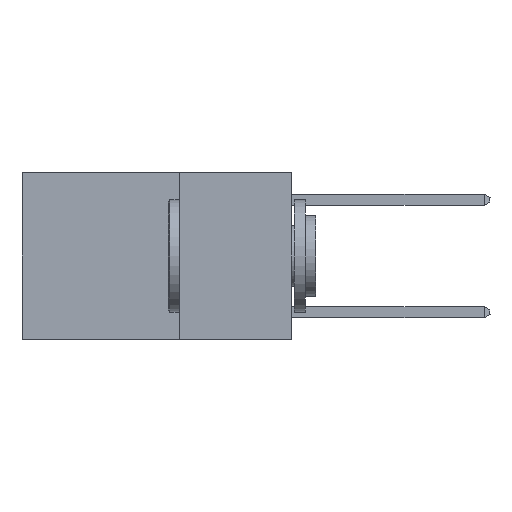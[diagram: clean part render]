
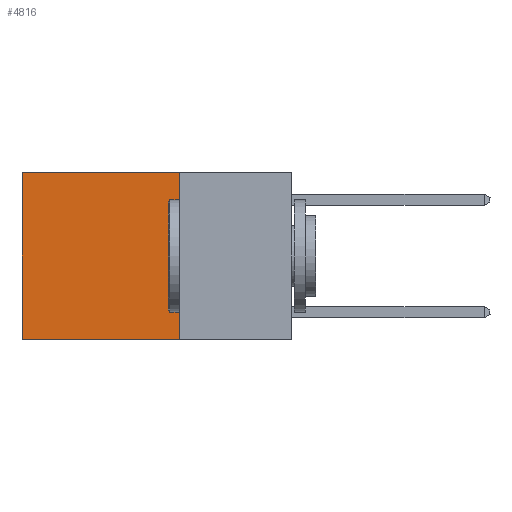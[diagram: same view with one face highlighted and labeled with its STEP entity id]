
A CAD part, left-side view. The second image highlights one B-rep face of the part: STEP entity #4816.
In plain terms, the highlighted planar face has unit normal (-1, 0, 0).
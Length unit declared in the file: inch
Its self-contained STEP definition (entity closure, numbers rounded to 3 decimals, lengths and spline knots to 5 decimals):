
#78 = LINE ( 'NONE', #3020, #11518 ) ;
#311 = CARTESIAN_POINT ( 'NONE',  ( 0.2625, 0.25, 0. ) ) ;
#857 = EDGE_CURVE ( 'NONE', #5635, #7671, #12639, .T. ) ;
#1300 = DIRECTION ( 'NONE',  ( 0., 0., -1. ) ) ;
#1972 = DIRECTION ( 'NONE',  ( 0., 0., -1. ) ) ;
#2301 = EDGE_LOOP ( 'NONE', ( #2913, #7093, #7404, #3521 ) ) ;
#2913 = ORIENTED_EDGE ( 'NONE', *, *, #4659, .T. ) ;
#3020 = CARTESIAN_POINT ( 'NONE',  ( 0.2625, 0.25, -0.37 ) ) ;
#3116 = CARTESIAN_POINT ( 'NONE',  ( 0.2625, 0.6, -0.37 ) ) ;
#3497 = VECTOR ( 'NONE', #10661, 39.37008 ) ;
#3521 = ORIENTED_EDGE ( 'NONE', *, *, #857, .T. ) ;
#4631 = DIRECTION ( 'NONE',  ( 1., 0., 0. ) ) ;
#4659 = EDGE_CURVE ( 'NONE', #7671, #6860, #12641, .T. ) ;
#4816 = ADVANCED_FACE ( 'NONE', ( #8830 ), #9019, .F. ) ;
#4895 = CARTESIAN_POINT ( 'NONE',  ( 0.2625, 0.25, -0.37 ) ) ;
#5111 = VECTOR ( 'NONE', #1972, 39.37008 ) ;
#5118 = LINE ( 'NONE', #9227, #5111 ) ;
#5635 = VERTEX_POINT ( 'NONE', #311 ) ;
#6021 = EDGE_CURVE ( 'NONE', #11185, #6860, #78, .T. ) ;
#6753 = DIRECTION ( 'NONE',  ( 0., 0., -1. ) ) ;
#6860 = VERTEX_POINT ( 'NONE', #3116 ) ;
#7093 = ORIENTED_EDGE ( 'NONE', *, *, #6021, .F. ) ;
#7309 = DIRECTION ( 'NONE',  ( 0., 1., 0. ) ) ;
#7404 = ORIENTED_EDGE ( 'NONE', *, *, #12106, .F. ) ;
#7671 = VERTEX_POINT ( 'NONE', #9993 ) ;
#7755 = CARTESIAN_POINT ( 'NONE',  ( 0.2625, 0.25, 0. ) ) ;
#8830 = FACE_OUTER_BOUND ( 'NONE', #2301, .T. ) ;
#9019 = PLANE ( 'NONE',  #9957 ) ;
#9227 = CARTESIAN_POINT ( 'NONE',  ( 0.2625, 0.25, 0. ) ) ;
#9511 = CARTESIAN_POINT ( 'NONE',  ( 0.2625, 0.6, 0. ) ) ;
#9957 = AXIS2_PLACEMENT_3D ( 'NONE', #7755, #4631, #6753 ) ;
#9993 = CARTESIAN_POINT ( 'NONE',  ( 0.2625, 0.6, 0. ) ) ;
#10661 = DIRECTION ( 'NONE',  ( 0., 1., 0. ) ) ;
#10730 = VECTOR ( 'NONE', #1300, 39.37008 ) ;
#11185 = VERTEX_POINT ( 'NONE', #4895 ) ;
#11471 = CARTESIAN_POINT ( 'NONE',  ( 0.2625, 0.25, 0. ) ) ;
#11518 = VECTOR ( 'NONE', #7309, 39.37008 ) ;
#12106 = EDGE_CURVE ( 'NONE', #5635, #11185, #5118, .T. ) ;
#12639 = LINE ( 'NONE', #11471, #3497 ) ;
#12641 = LINE ( 'NONE', #9511, #10730 ) ;
